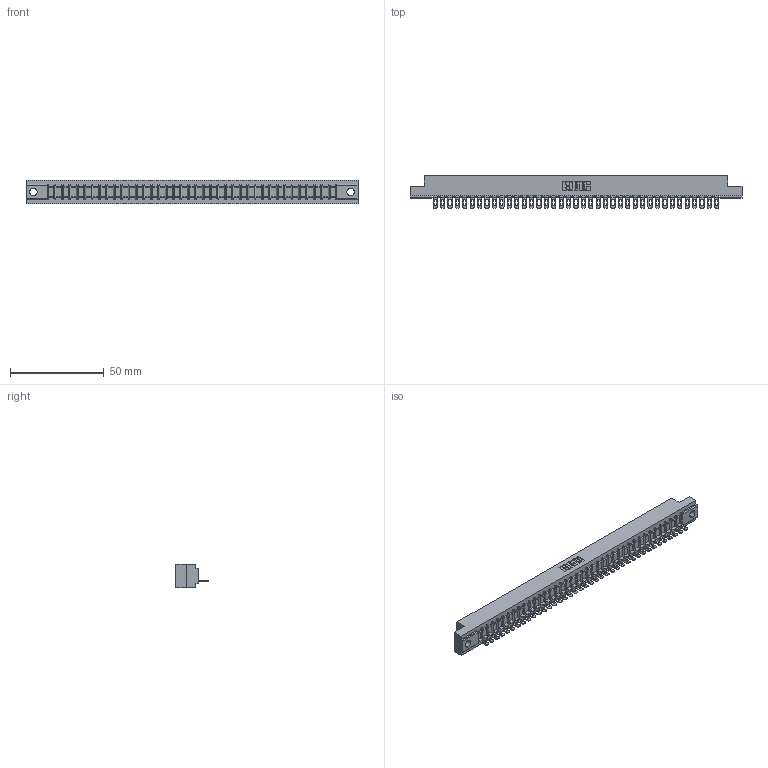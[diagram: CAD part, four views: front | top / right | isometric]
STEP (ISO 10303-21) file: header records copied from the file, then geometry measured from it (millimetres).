
FILE_DESCRIPTION (( 'STEP AP203' ), '1' );
FILE_NAME ('307-039-501-104.STEP', '2018-08-05T12:54:53', ( '' ), ( '' ), 'SwSTEP 2.0', 'SolidWorks 2016', '' );
FILE_SCHEMA (( 'CONFIG_CONTROL_DESIGN' ));
Length unit declared in the file: inch
Products named in the file (3): 307 Part_.156 Dia Mounting Holes; 307-290-002_501; 307-039-501-104
Assembly tree (40 placements, depth 2):
  307-039-501-104
    307 Part_.156 Dia Mounting Holes
    307-290-002_501  x39
Bounding box: 177.55 x 17.42 x 12.7 mm (x, y, z)
Volume: 18905.3 mm3; surface area: 23804.3 mm2
Topology: 40 solids, 40 shells, 3136 faces, 9641 edges, 6318 vertices
Faces by surface type: plane 1800, cylinder 1256, sphere 80
Entity records: 35016 total; most frequent: CARTESIAN_POINT 5910, ORIENTED_EDGE 5898, DIRECTION 5739, EDGE_CURVE 2949, LINE 2261, VECTOR 2261, VERTEX_POINT 1910, AXIS2_PLACEMENT_3D 1739
